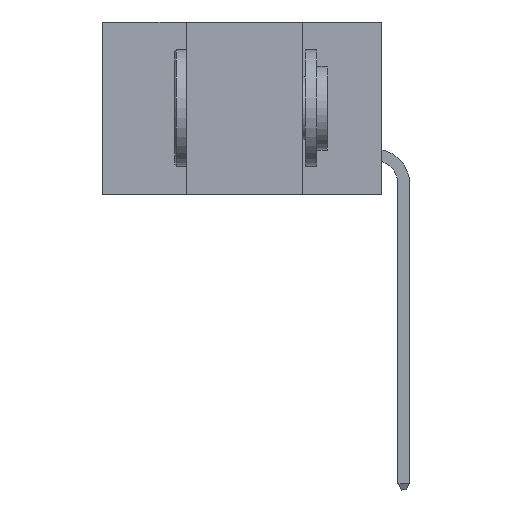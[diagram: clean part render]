
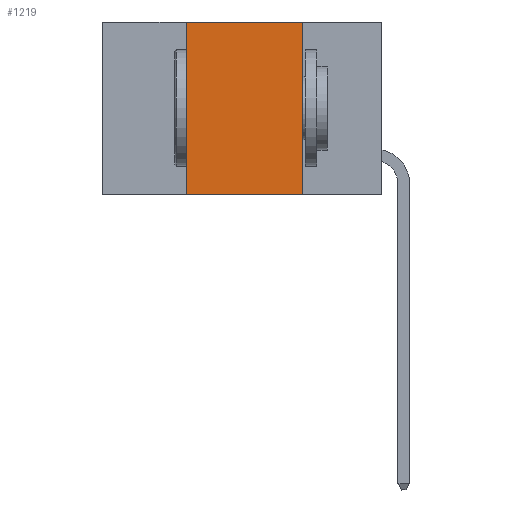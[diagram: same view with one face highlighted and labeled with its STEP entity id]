
A CAD part, left-side view. The second image highlights one B-rep face of the part: STEP entity #1219.
In plain terms, the highlighted planar face has unit normal (-1, 0, 0).
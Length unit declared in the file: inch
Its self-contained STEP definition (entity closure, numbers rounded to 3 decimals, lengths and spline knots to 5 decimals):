
#32 = DIRECTION ( 'NONE',  ( 0., 0., -1. ) ) ;
#1009 = EDGE_CURVE ( 'NONE', #1026, #6958, #7167, .T. ) ;
#1026 = VERTEX_POINT ( 'NONE', #17643 ) ;
#1219 = ADVANCED_FACE ( 'NONE', ( #2587 ), #1342, .F. ) ;
#1342 = PLANE ( 'NONE',  #10624 ) ;
#2450 = CARTESIAN_POINT ( 'NONE',  ( 0., 0.17, 0. ) ) ;
#2587 = FACE_OUTER_BOUND ( 'NONE', #9758, .T. ) ;
#3074 = CARTESIAN_POINT ( 'NONE',  ( 0., 0.42, 0. ) ) ;
#3591 = CARTESIAN_POINT ( 'NONE',  ( 0., 0.17, -0.37 ) ) ;
#5824 = ORIENTED_EDGE ( 'NONE', *, *, #10457, .F. ) ;
#6579 = VECTOR ( 'NONE', #10395, 39.37008 ) ;
#6958 = VERTEX_POINT ( 'NONE', #3591 ) ;
#7167 = LINE ( 'NONE', #8341, #6579 ) ;
#8306 = LINE ( 'NONE', #9604, #16904 ) ;
#8341 = CARTESIAN_POINT ( 'NONE',  ( 0., 0.6, -0.37 ) ) ;
#8891 = DIRECTION ( 'NONE',  ( 1., 0., 0. ) ) ;
#9604 = CARTESIAN_POINT ( 'NONE',  ( 0., 0.6, 0. ) ) ;
#9758 = EDGE_LOOP ( 'NONE', ( #12024, #5824, #16494, #10516 ) ) ;
#10395 = DIRECTION ( 'NONE',  ( 0., -1., 0. ) ) ;
#10457 = EDGE_CURVE ( 'NONE', #20543, #18070, #8306, .T. ) ;
#10516 = ORIENTED_EDGE ( 'NONE', *, *, #1009, .T. ) ;
#10624 = AXIS2_PLACEMENT_3D ( 'NONE', #19863, #8891, #12412 ) ;
#11045 = LINE ( 'NONE', #13153, #19394 ) ;
#12024 = ORIENTED_EDGE ( 'NONE', *, *, #16920, .F. ) ;
#12412 = DIRECTION ( 'NONE',  ( 0., 0., -1. ) ) ;
#12746 = CARTESIAN_POINT ( 'NONE',  ( 0., 0.17, 0. ) ) ;
#13153 = CARTESIAN_POINT ( 'NONE',  ( 0., 0.42, 0. ) ) ;
#16226 = LINE ( 'NONE', #2450, #22034 ) ;
#16494 = ORIENTED_EDGE ( 'NONE', *, *, #17247, .F. ) ;
#16904 = VECTOR ( 'NONE', #18463, 39.37008 ) ;
#16920 = EDGE_CURVE ( 'NONE', #18070, #6958, #16226, .T. ) ;
#17247 = EDGE_CURVE ( 'NONE', #1026, #20543, #11045, .T. ) ;
#17643 = CARTESIAN_POINT ( 'NONE',  ( 0., 0.42, -0.37 ) ) ;
#18070 = VERTEX_POINT ( 'NONE', #12746 ) ;
#18463 = DIRECTION ( 'NONE',  ( 0., -1., 0. ) ) ;
#18982 = DIRECTION ( 'NONE',  ( 0., 0., 1. ) ) ;
#19394 = VECTOR ( 'NONE', #18982, 39.37008 ) ;
#19863 = CARTESIAN_POINT ( 'NONE',  ( 0., 0.6, 0. ) ) ;
#20543 = VERTEX_POINT ( 'NONE', #3074 ) ;
#22034 = VECTOR ( 'NONE', #32, 39.37008 ) ;
